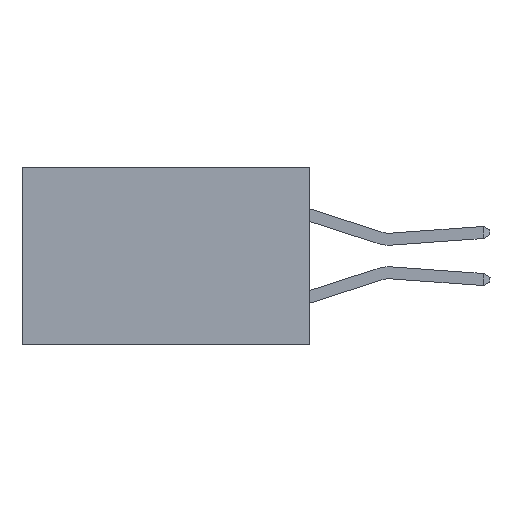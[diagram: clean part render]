
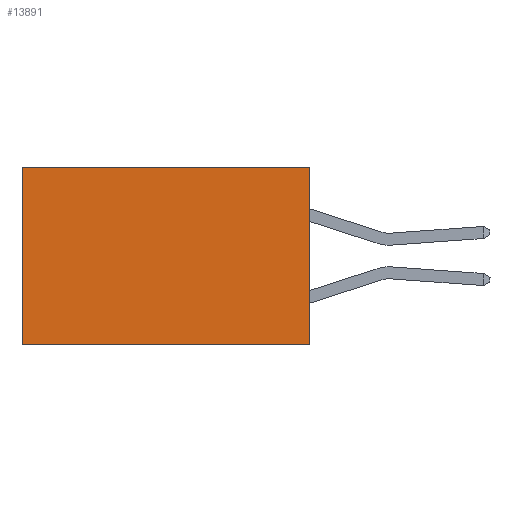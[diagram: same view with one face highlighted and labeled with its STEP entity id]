
A CAD part, left-side view. The second image highlights one B-rep face of the part: STEP entity #13891.
In plain terms, the highlighted planar face has unit normal (-1, 0, 0).
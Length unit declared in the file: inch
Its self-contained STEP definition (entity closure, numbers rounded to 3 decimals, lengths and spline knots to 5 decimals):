
#522 = EDGE_CURVE ( 'NONE', #7351, #3511, #2888, .T. ) ;
#1084 = DIRECTION ( 'NONE',  ( 0., 0., -1. ) ) ;
#2080 = CARTESIAN_POINT ( 'NONE',  ( 0.2615, 0., 0. ) ) ;
#2586 = VERTEX_POINT ( 'NONE', #8973 ) ;
#2884 = CARTESIAN_POINT ( 'NONE',  ( 0.2615, 0., -0.37 ) ) ;
#2888 = LINE ( 'NONE', #14853, #12856 ) ;
#2978 = CARTESIAN_POINT ( 'NONE',  ( 0.2615, 0., -0.37 ) ) ;
#3126 = LINE ( 'NONE', #2978, #23333 ) ;
#3511 = VERTEX_POINT ( 'NONE', #16678 ) ;
#3643 = EDGE_CURVE ( 'NONE', #6073, #2586, #20288, .T. ) ;
#4871 = DIRECTION ( 'NONE',  ( 1., 0., 0. ) ) ;
#6055 = CARTESIAN_POINT ( 'NONE',  ( 0.2615, 0.6, 0. ) ) ;
#6073 = VERTEX_POINT ( 'NONE', #2080 ) ;
#7351 = VERTEX_POINT ( 'NONE', #6055 ) ;
#8973 = CARTESIAN_POINT ( 'NONE',  ( 0.2615, 0., -0.37 ) ) ;
#9014 = DIRECTION ( 'NONE',  ( 0., 1., 0. ) ) ;
#9503 = VECTOR ( 'NONE', #13053, 39.37008 ) ;
#9714 = EDGE_CURVE ( 'NONE', #2586, #3511, #3126, .T. ) ;
#10105 = ORIENTED_EDGE ( 'NONE', *, *, #9714, .F. ) ;
#10120 = LINE ( 'NONE', #10973, #9503 ) ;
#10973 = CARTESIAN_POINT ( 'NONE',  ( 0.2615, 0., 0. ) ) ;
#12856 = VECTOR ( 'NONE', #1084, 39.37008 ) ;
#13053 = DIRECTION ( 'NONE',  ( 0., 1., 0. ) ) ;
#13612 = ORIENTED_EDGE ( 'NONE', *, *, #15328, .T. ) ;
#13891 = ADVANCED_FACE ( 'NONE', ( #22927 ), #14745, .F. ) ;
#14745 = PLANE ( 'NONE',  #15817 ) ;
#14784 = CARTESIAN_POINT ( 'NONE',  ( 0.2615, 0., -0.37 ) ) ;
#14853 = CARTESIAN_POINT ( 'NONE',  ( 0.2615, 0.6, -0.37 ) ) ;
#15328 = EDGE_CURVE ( 'NONE', #6073, #7351, #10120, .T. ) ;
#15817 = AXIS2_PLACEMENT_3D ( 'NONE', #2884, #4871, #18636 ) ;
#16321 = DIRECTION ( 'NONE',  ( 0., 0., -1. ) ) ;
#16678 = CARTESIAN_POINT ( 'NONE',  ( 0.2615, 0.6, -0.37 ) ) ;
#18636 = DIRECTION ( 'NONE',  ( 0., 0., -1. ) ) ;
#19682 = VECTOR ( 'NONE', #16321, 39.37008 ) ;
#20288 = LINE ( 'NONE', #14784, #19682 ) ;
#20538 = EDGE_LOOP ( 'NONE', ( #24659, #10105, #23199, #13612 ) ) ;
#22927 = FACE_OUTER_BOUND ( 'NONE', #20538, .T. ) ;
#23199 = ORIENTED_EDGE ( 'NONE', *, *, #3643, .F. ) ;
#23333 = VECTOR ( 'NONE', #9014, 39.37008 ) ;
#24659 = ORIENTED_EDGE ( 'NONE', *, *, #522, .T. ) ;
